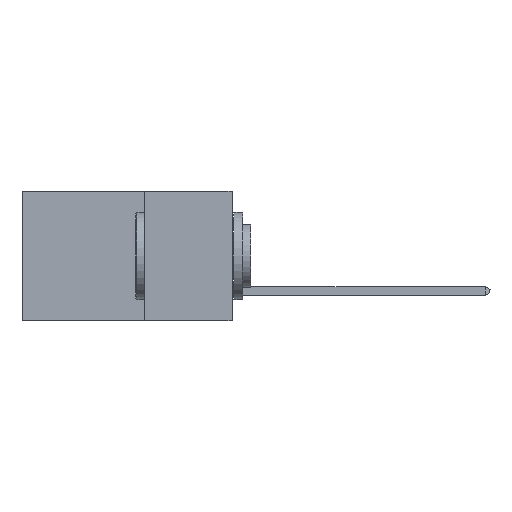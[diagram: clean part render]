
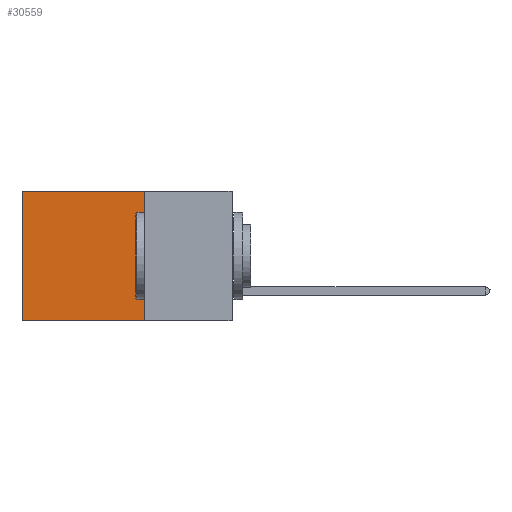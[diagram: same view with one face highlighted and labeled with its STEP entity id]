
A CAD part, left-side view. The second image highlights one B-rep face of the part: STEP entity #30559.
In plain terms, the highlighted planar face has unit normal (-1, 0, 0).
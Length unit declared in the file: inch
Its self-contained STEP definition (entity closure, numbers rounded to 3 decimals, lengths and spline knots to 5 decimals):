
#379 = DIRECTION ( 'NONE',  ( 1., 0., 0. ) ) ;
#3658 = CARTESIAN_POINT ( 'NONE',  ( 0.2875, 0.25, 0. ) ) ;
#3753 = VECTOR ( 'NONE', #35124, 39.37008 ) ;
#7608 = DIRECTION ( 'NONE',  ( 0., 0., -1. ) ) ;
#8550 = DIRECTION ( 'NONE',  ( 0., 0., -1. ) ) ;
#8952 = VECTOR ( 'NONE', #8550, 39.37008 ) ;
#10078 = CARTESIAN_POINT ( 'NONE',  ( 0.2875, 0.6, 0. ) ) ;
#11406 = LINE ( 'NONE', #10078, #34491 ) ;
#13056 = VERTEX_POINT ( 'NONE', #35878 ) ;
#13451 = VECTOR ( 'NONE', #39469, 39.37008 ) ;
#15115 = CARTESIAN_POINT ( 'NONE',  ( 0.2875, 0.25, 0. ) ) ;
#15581 = VERTEX_POINT ( 'NONE', #33126 ) ;
#15806 = EDGE_CURVE ( 'NONE', #13056, #15581, #22513, .T. ) ;
#17386 = LINE ( 'NONE', #15115, #8952 ) ;
#17453 = FACE_OUTER_BOUND ( 'NONE', #29451, .T. ) ;
#18937 = LINE ( 'NONE', #30025, #13451 ) ;
#19282 = CARTESIAN_POINT ( 'NONE',  ( 0.2875, 0.25, 0. ) ) ;
#21674 = CARTESIAN_POINT ( 'NONE',  ( 0.2875, 0.25, -0.37 ) ) ;
#22156 = VERTEX_POINT ( 'NONE', #21674 ) ;
#22334 = DIRECTION ( 'NONE',  ( 0., 0., -1. ) ) ;
#22513 = LINE ( 'NONE', #3658, #3753 ) ;
#23451 = EDGE_CURVE ( 'NONE', #22156, #27000, #18937, .T. ) ;
#25131 = EDGE_CURVE ( 'NONE', #13056, #22156, #17386, .T. ) ;
#25446 = ORIENTED_EDGE ( 'NONE', *, *, #26165, .T. ) ;
#26165 = EDGE_CURVE ( 'NONE', #15581, #27000, #11406, .T. ) ;
#27000 = VERTEX_POINT ( 'NONE', #38860 ) ;
#28638 = PLANE ( 'NONE',  #38349 ) ;
#29364 = ORIENTED_EDGE ( 'NONE', *, *, #23451, .F. ) ;
#29451 = EDGE_LOOP ( 'NONE', ( #25446, #29364, #37185, #37912 ) ) ;
#30025 = CARTESIAN_POINT ( 'NONE',  ( 0.2875, 0.25, -0.37 ) ) ;
#30559 = ADVANCED_FACE ( 'NONE', ( #17453 ), #28638, .F. ) ;
#33126 = CARTESIAN_POINT ( 'NONE',  ( 0.2875, 0.6, 0. ) ) ;
#34491 = VECTOR ( 'NONE', #7608, 39.37008 ) ;
#35124 = DIRECTION ( 'NONE',  ( 0., 1., 0. ) ) ;
#35878 = CARTESIAN_POINT ( 'NONE',  ( 0.2875, 0.25, 0. ) ) ;
#37185 = ORIENTED_EDGE ( 'NONE', *, *, #25131, .F. ) ;
#37912 = ORIENTED_EDGE ( 'NONE', *, *, #15806, .T. ) ;
#38349 = AXIS2_PLACEMENT_3D ( 'NONE', #19282, #379, #22334 ) ;
#38860 = CARTESIAN_POINT ( 'NONE',  ( 0.2875, 0.6, -0.37 ) ) ;
#39469 = DIRECTION ( 'NONE',  ( 0., 1., 0. ) ) ;
